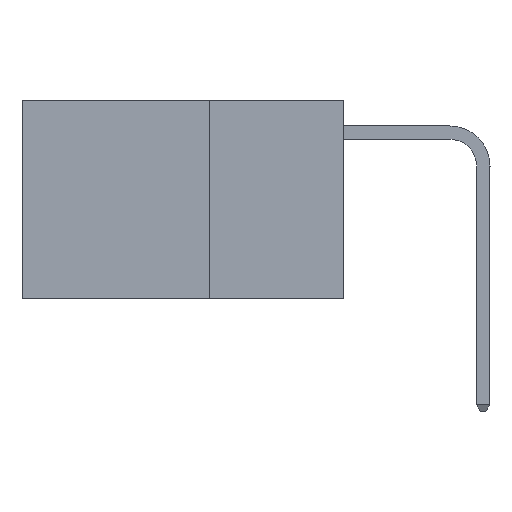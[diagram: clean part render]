
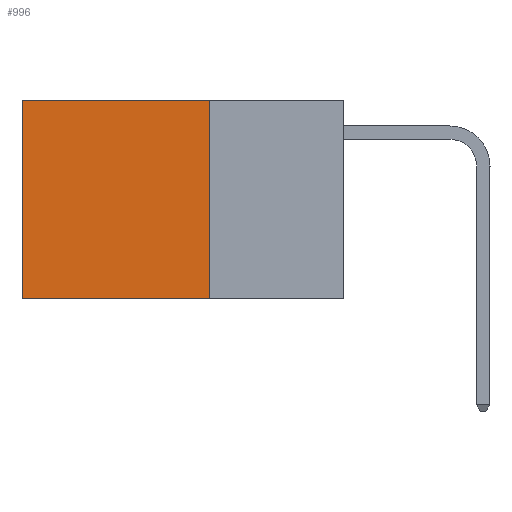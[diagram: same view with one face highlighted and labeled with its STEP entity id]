
A CAD part, left-side view. The second image highlights one B-rep face of the part: STEP entity #996.
In plain terms, the highlighted planar face has unit normal (-1, 0, 0).
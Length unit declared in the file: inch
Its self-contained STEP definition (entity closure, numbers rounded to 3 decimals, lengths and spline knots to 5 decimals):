
#36 = VERTEX_POINT ( 'NONE', #9529 ) ;
#103 = EDGE_LOOP ( 'NONE', ( #8775, #1625, #7487, #9379 ) ) ;
#240 = VECTOR ( 'NONE', #4471, 39.37008 ) ;
#433 = VECTOR ( 'NONE', #8878, 39.37008 ) ;
#750 = LINE ( 'NONE', #6945, #433 ) ;
#996 = ADVANCED_FACE ( 'NONE', ( #3825 ), #3485, .F. ) ;
#1625 = ORIENTED_EDGE ( 'NONE', *, *, #9245, .F. ) ;
#1634 = VECTOR ( 'NONE', #9183, 39.37008 ) ;
#2515 = CARTESIAN_POINT ( 'NONE',  ( 0.2625, 0.25, 0. ) ) ;
#3485 = PLANE ( 'NONE',  #6229 ) ;
#3825 = FACE_OUTER_BOUND ( 'NONE', #103, .T. ) ;
#4319 = EDGE_CURVE ( 'NONE', #8881, #7491, #750, .T. ) ;
#4471 = DIRECTION ( 'NONE',  ( 0., 0., -1. ) ) ;
#4587 = LINE ( 'NONE', #10941, #1634 ) ;
#6229 = AXIS2_PLACEMENT_3D ( 'NONE', #2515, #9742, #6866 ) ;
#6547 = CARTESIAN_POINT ( 'NONE',  ( 0.2625, 0.25, 0. ) ) ;
#6866 = DIRECTION ( 'NONE',  ( 0., 0., -1. ) ) ;
#6945 = CARTESIAN_POINT ( 'NONE',  ( 0.2625, 0.6, 0. ) ) ;
#7168 = EDGE_CURVE ( 'NONE', #10851, #8881, #8796, .T. ) ;
#7487 = ORIENTED_EDGE ( 'NONE', *, *, #8714, .F. ) ;
#7491 = VERTEX_POINT ( 'NONE', #8427 ) ;
#8065 = LINE ( 'NONE', #10985, #240 ) ;
#8427 = CARTESIAN_POINT ( 'NONE',  ( 0.2625, 0.6, -0.37 ) ) ;
#8524 = CARTESIAN_POINT ( 'NONE',  ( 0.2625, 0.6, 0. ) ) ;
#8714 = EDGE_CURVE ( 'NONE', #10851, #36, #8065, .T. ) ;
#8775 = ORIENTED_EDGE ( 'NONE', *, *, #4319, .T. ) ;
#8796 = LINE ( 'NONE', #6547, #9086 ) ;
#8878 = DIRECTION ( 'NONE',  ( 0., 0., -1. ) ) ;
#8881 = VERTEX_POINT ( 'NONE', #8524 ) ;
#9086 = VECTOR ( 'NONE', #11991, 39.37008 ) ;
#9183 = DIRECTION ( 'NONE',  ( 0., 1., 0. ) ) ;
#9245 = EDGE_CURVE ( 'NONE', #36, #7491, #4587, .T. ) ;
#9379 = ORIENTED_EDGE ( 'NONE', *, *, #7168, .T. ) ;
#9529 = CARTESIAN_POINT ( 'NONE',  ( 0.2625, 0.25, -0.37 ) ) ;
#9742 = DIRECTION ( 'NONE',  ( 1., 0., 0. ) ) ;
#10054 = CARTESIAN_POINT ( 'NONE',  ( 0.2625, 0.25, 0. ) ) ;
#10851 = VERTEX_POINT ( 'NONE', #10054 ) ;
#10941 = CARTESIAN_POINT ( 'NONE',  ( 0.2625, 0.25, -0.37 ) ) ;
#10985 = CARTESIAN_POINT ( 'NONE',  ( 0.2625, 0.25, 0. ) ) ;
#11991 = DIRECTION ( 'NONE',  ( 0., 1., 0. ) ) ;
